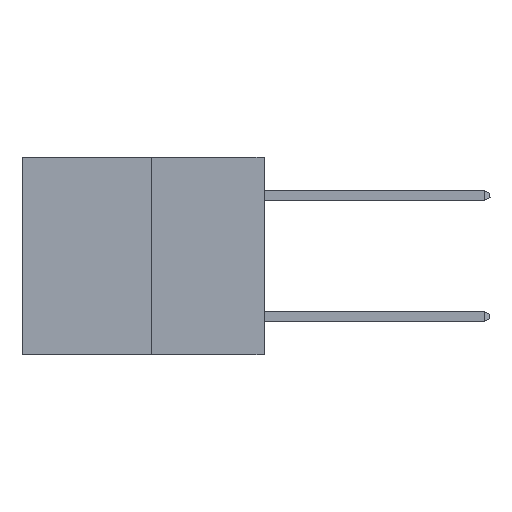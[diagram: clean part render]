
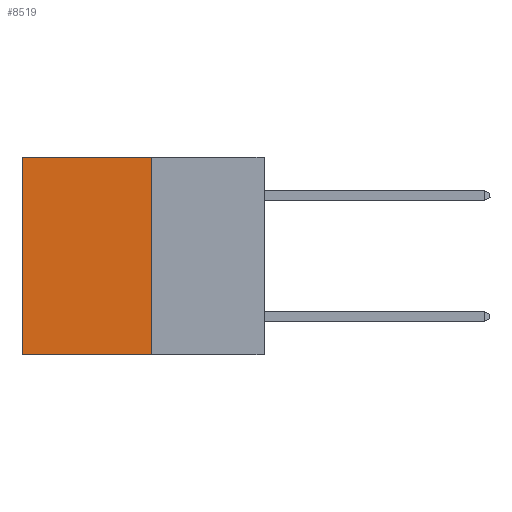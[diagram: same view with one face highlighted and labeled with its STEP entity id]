
A CAD part, left-side view. The second image highlights one B-rep face of the part: STEP entity #8519.
In plain terms, the highlighted planar face has unit normal (-1, 0, 0).
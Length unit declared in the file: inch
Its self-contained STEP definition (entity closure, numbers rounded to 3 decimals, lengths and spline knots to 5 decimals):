
#245 = VERTEX_POINT ( 'NONE', #4871 ) ;
#256 = CARTESIAN_POINT ( 'NONE',  ( 0.3165, 0.6, -0.49 ) ) ;
#843 = CARTESIAN_POINT ( 'NONE',  ( 0.3165, 0.28, -0.49 ) ) ;
#2497 = DIRECTION ( 'NONE',  ( 0., 0., -1. ) ) ;
#2805 = DIRECTION ( 'NONE',  ( 0., 0., -1. ) ) ;
#3282 = PLANE ( 'NONE',  #20881 ) ;
#4134 = LINE ( 'NONE', #843, #10585 ) ;
#4561 = VECTOR ( 'NONE', #19469, 39.37008 ) ;
#4803 = CARTESIAN_POINT ( 'NONE',  ( 0.3165, 0.28, -0.49 ) ) ;
#4871 = CARTESIAN_POINT ( 'NONE',  ( 0.3165, 0.6, 0. ) ) ;
#5406 = LINE ( 'NONE', #4803, #4561 ) ;
#5847 = EDGE_CURVE ( 'NONE', #6839, #13760, #4134, .T. ) ;
#6839 = VERTEX_POINT ( 'NONE', #16896 ) ;
#6901 = ORIENTED_EDGE ( 'NONE', *, *, #9760, .T. ) ;
#7205 = CARTESIAN_POINT ( 'NONE',  ( 0.3165, 0.28, -0.49 ) ) ;
#8269 = LINE ( 'NONE', #256, #18411 ) ;
#8519 = ADVANCED_FACE ( 'NONE', ( #18320 ), #3282, .F. ) ;
#9178 = CARTESIAN_POINT ( 'NONE',  ( 0.3165, 0.28, -0.49 ) ) ;
#9304 = CARTESIAN_POINT ( 'NONE',  ( 0.3165, 0.6, -0.49 ) ) ;
#9760 = EDGE_CURVE ( 'NONE', #6839, #245, #16788, .T. ) ;
#10363 = ORIENTED_EDGE ( 'NONE', *, *, #21737, .F. ) ;
#10585 = VECTOR ( 'NONE', #2805, 39.37008 ) ;
#11659 = EDGE_CURVE ( 'NONE', #245, #21693, #8269, .T. ) ;
#13760 = VERTEX_POINT ( 'NONE', #9178 ) ;
#16430 = DIRECTION ( 'NONE',  ( 1., 0., 0. ) ) ;
#16788 = LINE ( 'NONE', #22903, #22776 ) ;
#16896 = CARTESIAN_POINT ( 'NONE',  ( 0.3165, 0.28, 0. ) ) ;
#17752 = EDGE_LOOP ( 'NONE', ( #17834, #10363, #20564, #6901 ) ) ;
#17834 = ORIENTED_EDGE ( 'NONE', *, *, #11659, .T. ) ;
#18320 = FACE_OUTER_BOUND ( 'NONE', #17752, .T. ) ;
#18411 = VECTOR ( 'NONE', #2497, 39.37008 ) ;
#19286 = DIRECTION ( 'NONE',  ( 0., 1., 0. ) ) ;
#19469 = DIRECTION ( 'NONE',  ( 0., 1., 0. ) ) ;
#20564 = ORIENTED_EDGE ( 'NONE', *, *, #5847, .F. ) ;
#20881 = AXIS2_PLACEMENT_3D ( 'NONE', #7205, #16430, #21739 ) ;
#21693 = VERTEX_POINT ( 'NONE', #9304 ) ;
#21737 = EDGE_CURVE ( 'NONE', #13760, #21693, #5406, .T. ) ;
#21739 = DIRECTION ( 'NONE',  ( 0., 0., -1. ) ) ;
#22776 = VECTOR ( 'NONE', #19286, 39.37008 ) ;
#22903 = CARTESIAN_POINT ( 'NONE',  ( 0.3165, 0.28, 0. ) ) ;
